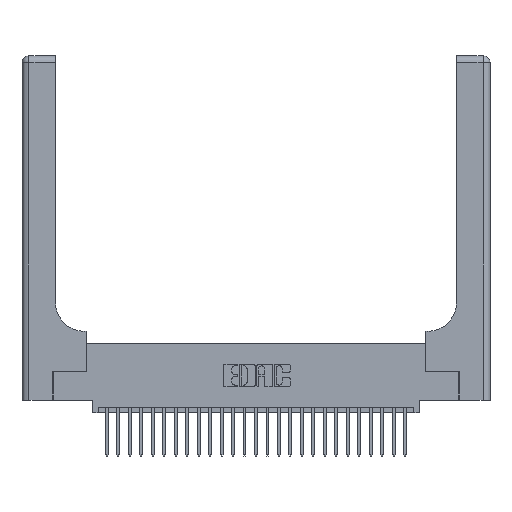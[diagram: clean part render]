
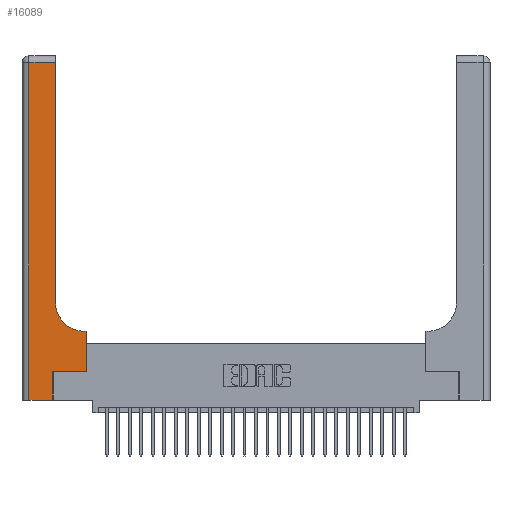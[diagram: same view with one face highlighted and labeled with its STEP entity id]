
A CAD part, top view. The second image highlights one B-rep face of the part: STEP entity #16089.
In plain terms, the highlighted planar face has unit normal (0, 0, 1).
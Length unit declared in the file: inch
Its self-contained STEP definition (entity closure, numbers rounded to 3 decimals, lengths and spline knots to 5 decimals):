
#329 = LINE ( 'NONE', #23740, #5563 ) ;
#1010 = DIRECTION ( 'NONE',  ( 0., 0., -1. ) ) ;
#1314 = CARTESIAN_POINT ( 'NONE',  ( 0.2915, 0.85, 0.37 ) ) ;
#1606 = VECTOR ( 'NONE', #6680, 39.37008 ) ;
#1711 = DIRECTION ( 'NONE',  ( 0., 1., 0. ) ) ;
#1875 = DIRECTION ( 'NONE',  ( 0., 1., 0. ) ) ;
#2131 = EDGE_CURVE ( 'NONE', #18768, #23847, #329, .T. ) ;
#2941 = ORIENTED_EDGE ( 'NONE', *, *, #11809, .T. ) ;
#2942 = EDGE_CURVE ( 'NONE', #25459, #6710, #3805, .T. ) ;
#2992 = VERTEX_POINT ( 'NONE', #4137 ) ;
#3526 = DIRECTION ( 'NONE',  ( 1., 0., 0. ) ) ;
#3636 = CARTESIAN_POINT ( 'NONE',  ( 0.269, 0.25, 0.37 ) ) ;
#3805 = LINE ( 'NONE', #10535, #19920 ) ;
#4137 = CARTESIAN_POINT ( 'NONE',  ( 0.06, 0., 0.37 ) ) ;
#5231 = FACE_OUTER_BOUND ( 'NONE', #12047, .T. ) ;
#5280 = CARTESIAN_POINT ( 'NONE',  ( 0.269, 0., 0.37 ) ) ;
#5563 = VECTOR ( 'NONE', #23587, 39.37008 ) ;
#5950 = CARTESIAN_POINT ( 'NONE',  ( 0.5585, 0.6, 0.37 ) ) ;
#5951 = ORIENTED_EDGE ( 'NONE', *, *, #11971, .T. ) ;
#6149 = CARTESIAN_POINT ( 'NONE',  ( 0.5415, 0.85, 0.37 ) ) ;
#6320 = LINE ( 'NONE', #27585, #27616 ) ;
#6680 = DIRECTION ( 'NONE',  ( -1., 0., 0. ) ) ;
#6710 = VERTEX_POINT ( 'NONE', #5950 ) ;
#7358 = EDGE_CURVE ( 'NONE', #2992, #11693, #24170, .T. ) ;
#7447 = ORIENTED_EDGE ( 'NONE', *, *, #7358, .T. ) ;
#7807 = DIRECTION ( 'NONE',  ( -1., 0., 0. ) ) ;
#7832 = CARTESIAN_POINT ( 'NONE',  ( 0.269, 0.25, 0.37 ) ) ;
#8380 = DIRECTION ( 'NONE',  ( 1., 0., 0. ) ) ;
#8727 = LINE ( 'NONE', #10059, #25502 ) ;
#9238 = VERTEX_POINT ( 'NONE', #3636 ) ;
#9386 = EDGE_CURVE ( 'NONE', #11693, #9238, #23225, .T. ) ;
#10059 = CARTESIAN_POINT ( 'NONE',  ( 0., 2.94, 0.37 ) ) ;
#10535 = CARTESIAN_POINT ( 'NONE',  ( 0.5585, 0.25, 0.37 ) ) ;
#10612 = ORIENTED_EDGE ( 'NONE', *, *, #18287, .T. ) ;
#11257 = EDGE_CURVE ( 'NONE', #15997, #2992, #6320, .T. ) ;
#11693 = VERTEX_POINT ( 'NONE', #5280 ) ;
#11809 = EDGE_CURVE ( 'NONE', #23847, #15997, #8727, .T. ) ;
#11971 = EDGE_CURVE ( 'NONE', #14794, #18768, #22719, .T. ) ;
#11992 = AXIS2_PLACEMENT_3D ( 'NONE', #27357, #1010, #16457 ) ;
#12047 = EDGE_LOOP ( 'NONE', ( #18369, #2941, #14322, #7447, #15040, #10612, #19131, #23380, #5951 ) ) ;
#12543 = VECTOR ( 'NONE', #3526, 39.37008 ) ;
#13733 = LINE ( 'NONE', #7832, #24673 ) ;
#14230 = PLANE ( 'NONE',  #11992 ) ;
#14322 = ORIENTED_EDGE ( 'NONE', *, *, #11257, .T. ) ;
#14458 = DIRECTION ( 'NONE',  ( 0., -1., 0. ) ) ;
#14794 = VERTEX_POINT ( 'NONE', #18026 ) ;
#15040 = ORIENTED_EDGE ( 'NONE', *, *, #9386, .T. ) ;
#15449 = CARTESIAN_POINT ( 'NONE',  ( 0.2915, 0.6, 0.37 ) ) ;
#15997 = VERTEX_POINT ( 'NONE', #22613 ) ;
#16089 = ADVANCED_FACE ( 'NONE', ( #5231 ), #14230, .F. ) ;
#16457 = DIRECTION ( 'NONE',  ( -1., 0., 0. ) ) ;
#17265 = CARTESIAN_POINT ( 'NONE',  ( 0.269, 0., 0.37 ) ) ;
#17419 = VECTOR ( 'NONE', #1875, 39.37008 ) ;
#18026 = CARTESIAN_POINT ( 'NONE',  ( 0.5415, 0.6, 0.37 ) ) ;
#18287 = EDGE_CURVE ( 'NONE', #9238, #25459, #13733, .T. ) ;
#18369 = ORIENTED_EDGE ( 'NONE', *, *, #2131, .T. ) ;
#18768 = VERTEX_POINT ( 'NONE', #1314 ) ;
#18867 = CARTESIAN_POINT ( 'NONE',  ( 0., 0., 0.37 ) ) ;
#19131 = ORIENTED_EDGE ( 'NONE', *, *, #2942, .T. ) ;
#19145 = LINE ( 'NONE', #15449, #1606 ) ;
#19535 = AXIS2_PLACEMENT_3D ( 'NONE', #6149, #21472, #8380 ) ;
#19691 = EDGE_CURVE ( 'NONE', #6710, #14794, #19145, .T. ) ;
#19920 = VECTOR ( 'NONE', #1711, 39.37008 ) ;
#20884 = CARTESIAN_POINT ( 'NONE',  ( 0.5585, 0.25, 0.37 ) ) ;
#21472 = DIRECTION ( 'NONE',  ( 0., 0., -1. ) ) ;
#22613 = CARTESIAN_POINT ( 'NONE',  ( 0.06, 2.94, 0.37 ) ) ;
#22719 = CIRCLE ( 'NONE', #19535, 0.25 ) ;
#23124 = DIRECTION ( 'NONE',  ( 1., 0., 0. ) ) ;
#23225 = LINE ( 'NONE', #17265, #17419 ) ;
#23380 = ORIENTED_EDGE ( 'NONE', *, *, #19691, .T. ) ;
#23587 = DIRECTION ( 'NONE',  ( 0., 1., 0. ) ) ;
#23740 = CARTESIAN_POINT ( 'NONE',  ( 0.2915, 3., 0.37 ) ) ;
#23847 = VERTEX_POINT ( 'NONE', #23848 ) ;
#23848 = CARTESIAN_POINT ( 'NONE',  ( 0.2915, 2.94, 0.37 ) ) ;
#24170 = LINE ( 'NONE', #18867, #12543 ) ;
#24673 = VECTOR ( 'NONE', #23124, 39.37008 ) ;
#25459 = VERTEX_POINT ( 'NONE', #20884 ) ;
#25502 = VECTOR ( 'NONE', #7807, 39.37008 ) ;
#27357 = CARTESIAN_POINT ( 'NONE',  ( 0., 3., 0.37 ) ) ;
#27585 = CARTESIAN_POINT ( 'NONE',  ( 0.06, 3., 0.37 ) ) ;
#27616 = VECTOR ( 'NONE', #14458, 39.37008 ) ;
